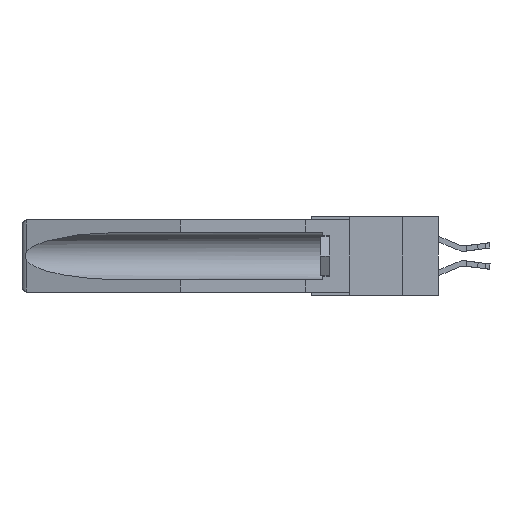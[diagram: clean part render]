
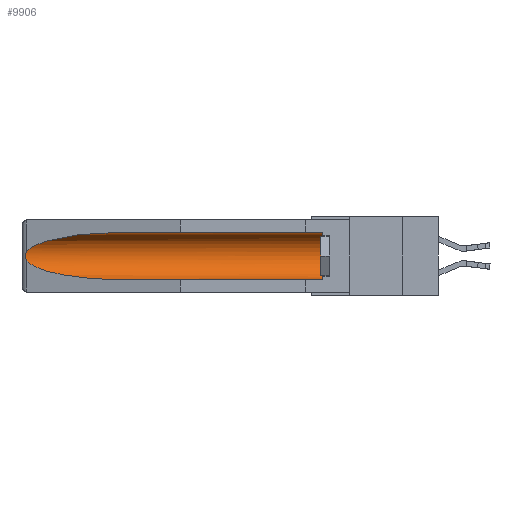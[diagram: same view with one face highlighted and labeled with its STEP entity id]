
A CAD part, left-side view. The second image highlights one B-rep face of the part: STEP entity #9906.
In plain terms, the highlighted cylindrical face has radius 2.857 mm (diameter 5.715 mm), a partial arc.
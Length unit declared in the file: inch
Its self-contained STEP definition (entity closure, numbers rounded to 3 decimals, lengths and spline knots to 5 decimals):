
#34 = CARTESIAN_POINT ( 'NONE',  ( 0.21114, 1.30732, -0.059 ) ) ;
#233 = EDGE_LOOP ( 'NONE', ( #16036, #12658, #5963, #11536, #10463, #13329 ) ) ;
#912 = CARTESIAN_POINT ( 'NONE',  ( 0.26537, 1.52718, -0.14972 ) ) ;
#1030 = DIRECTION ( 'NONE',  ( 0., -1., 0. ) ) ;
#1086 = CARTESIAN_POINT ( 'NONE',  ( 0.25451, 1.48313, -0.24835 ) ) ;
#1576 = VERTEX_POINT ( 'NONE', #9291 ) ;
#2275 = CARTESIAN_POINT ( 'NONE',  ( 0.155, 1.07973, -0.284 ) ) ;
#2370 = CIRCLE ( 'NONE', #5041, 0.1125 ) ;
#2386 = LINE ( 'NONE', #11219, #3428 ) ;
#2489 = CARTESIAN_POINT ( 'NONE',  ( 0.155, 0.126, -0.284 ) ) ;
#2666 = CARTESIAN_POINT ( 'NONE',  ( 0.2673, 1.5327, -0.16383 ) ) ;
#2679 = LINE ( 'NONE', #2741, #8973 ) ;
#2741 = CARTESIAN_POINT ( 'NONE',  ( 0.155, -0.30754, -0.284 ) ) ;
#2837 = VERTEX_POINT ( 'NONE', #912 ) ;
#3428 = VECTOR ( 'NONE', #12543, 39.37008 ) ;
#3486 = FACE_OUTER_BOUND ( 'NONE', #233, .T. ) ;
#3731 = CARTESIAN_POINT ( 'NONE',  ( 0.26537, 1.52718, -0.19328 ) ) ;
#4083 = EDGE_CURVE ( 'NONE', #2837, #1576, #13498, .T. ) ;
#4822 = CARTESIAN_POINT ( 'NONE',  ( 0.155, 0.126, -0.1715 ) ) ;
#4977 = EDGE_CURVE ( 'NONE', #15372, #9104, #2386, .T. ) ;
#5041 = AXIS2_PLACEMENT_3D ( 'NONE', #4822, #1030, #10107 ) ;
#5052 = CARTESIAN_POINT ( 'NONE',  ( 0.155, -0.30754, -0.1715 ) ) ;
#5107 = CARTESIAN_POINT ( 'NONE',  ( 0.21114, 1.30732, -0.284 ) ) ;
#5225 = DIRECTION ( 'NONE',  ( 0., 1., 0. ) ) ;
#5607 = CARTESIAN_POINT ( 'NONE',  ( 0.25451, 1.48313, -0.09465 ) ) ;
#5963 = ORIENTED_EDGE ( 'NONE', *, *, #8022, .T. ) ;
#6231 = DIRECTION ( 'NONE',  ( 0., 0., 1. ) ) ;
#6326 = CARTESIAN_POINT ( 'NONE',  ( 0.155, 1.07973, -0.059 ) ) ;
#6498 = CARTESIAN_POINT ( 'NONE',  ( 0.155, 1.07973, -0.284 ) ) ;
#6514 = CARTESIAN_POINT ( 'NONE',  ( 0.26597, 1.5296, -0.19026 ) ) ;
#6517 = DIRECTION ( 'NONE',  ( 0., 1., 0. ) ) ;
#6563 = CARTESIAN_POINT ( 'NONE',  ( 0.2675, 1.53308, -0.16763 ) ) ;
#6899 = CARTESIAN_POINT ( 'NONE',  ( 0.26537, 1.52718, -0.19328 ) ) ;
#7066 = EDGE_CURVE ( 'NONE', #9104, #2837, #16511, .T. ) ;
#8022 = EDGE_CURVE ( 'NONE', #1576, #14291, #14567, .T. ) ;
#8242 = CARTESIAN_POINT ( 'NONE',  ( 0.26655, 1.53094, -0.18657 ) ) ;
#8973 = VECTOR ( 'NONE', #6517, 39.37008 ) ;
#9087 = CARTESIAN_POINT ( 'NONE',  ( 0.26537, 1.52718, -0.14972 ) ) ;
#9104 = VERTEX_POINT ( 'NONE', #13728 ) ;
#9291 = CARTESIAN_POINT ( 'NONE',  ( 0.26537, 1.52718, -0.19328 ) ) ;
#9906 = ADVANCED_FACE ( 'NONE', ( #3486 ), #11087, .F. ) ;
#10107 = DIRECTION ( 'NONE',  ( 0., 0., 1. ) ) ;
#10389 = CARTESIAN_POINT ( 'NONE',  ( 0.26597, 1.52961, -0.15275 ) ) ;
#10446 = CARTESIAN_POINT ( 'NONE',  ( 0.26654, 1.53092, -0.15636 ) ) ;
#10463 = ORIENTED_EDGE ( 'NONE', *, *, #16157, .T. ) ;
#10783 = CARTESIAN_POINT ( 'NONE',  ( 0.2675, 1.53308, -0.17534 ) ) ;
#11087 = CYLINDRICAL_SURFACE ( 'NONE', #15756, 0.1125 ) ;
#11219 = CARTESIAN_POINT ( 'NONE',  ( 0.155, -0.30754, -0.059 ) ) ;
#11536 = ORIENTED_EDGE ( 'NONE', *, *, #13462, .F. ) ;
#12543 = DIRECTION ( 'NONE',  ( 0., 1., 0. ) ) ;
#12658 = ORIENTED_EDGE ( 'NONE', *, *, #4083, .T. ) ;
#13329 = ORIENTED_EDGE ( 'NONE', *, *, #4977, .T. ) ;
#13462 = EDGE_CURVE ( 'NONE', #16221, #14291, #2679, .T. ) ;
#13498 = B_SPLINE_CURVE_WITH_KNOTS ( 'NONE', 3,
 ( #9087, #10389, #10446, #2666, #6563, #10783, #14333, #8242, #6514, #6899 ),
 .UNSPECIFIED., .F., .F.,
 ( 4, 2, 2, 2, 4 ),
 ( 0., 0.00029, 0.00058, 0.00087, 0.00117 ),
 .UNSPECIFIED. ) ;
#13700 = CARTESIAN_POINT ( 'NONE',  ( 0.155, 0.126, -0.059 ) ) ;
#13728 = CARTESIAN_POINT ( 'NONE',  ( 0.155, 1.07973, -0.059 ) ) ;
#14291 = VERTEX_POINT ( 'NONE', #2275 ) ;
#14333 = CARTESIAN_POINT ( 'NONE',  ( 0.2673, 1.53269, -0.17917 ) ) ;
#14567 =( BOUNDED_CURVE ( )  B_SPLINE_CURVE ( 3, ( #3731, #1086, #5107, #6498 ),
 .UNSPECIFIED., .F., .F. ) 
 B_SPLINE_CURVE_WITH_KNOTS ( ( 4, 4 ),
 ( 0.1948, 1.5708 ),
 .UNSPECIFIED. ) 
 CURVE ( )  GEOMETRIC_REPRESENTATION_ITEM ( )  RATIONAL_B_SPLINE_CURVE ( ( 1., 0.848, 0.848, 1. ) ) 
 REPRESENTATION_ITEM ( '' )  );
#14703 = CARTESIAN_POINT ( 'NONE',  ( 0.26537, 1.52718, -0.14972 ) ) ;
#15372 = VERTEX_POINT ( 'NONE', #13700 ) ;
#15756 = AXIS2_PLACEMENT_3D ( 'NONE', #5052, #5225, #6231 ) ;
#16036 = ORIENTED_EDGE ( 'NONE', *, *, #7066, .T. ) ;
#16157 = EDGE_CURVE ( 'NONE', #16221, #15372, #2370, .T. ) ;
#16221 = VERTEX_POINT ( 'NONE', #2489 ) ;
#16511 =( BOUNDED_CURVE ( )  B_SPLINE_CURVE ( 3, ( #6326, #34, #5607, #14703 ),
 .UNSPECIFIED., .F., .F. ) 
 B_SPLINE_CURVE_WITH_KNOTS ( ( 4, 4 ),
 ( 4.71239, 6.08839 ),
 .UNSPECIFIED. ) 
 CURVE ( )  GEOMETRIC_REPRESENTATION_ITEM ( )  RATIONAL_B_SPLINE_CURVE ( ( 1., 0.848, 0.848, 1. ) ) 
 REPRESENTATION_ITEM ( '' )  );
